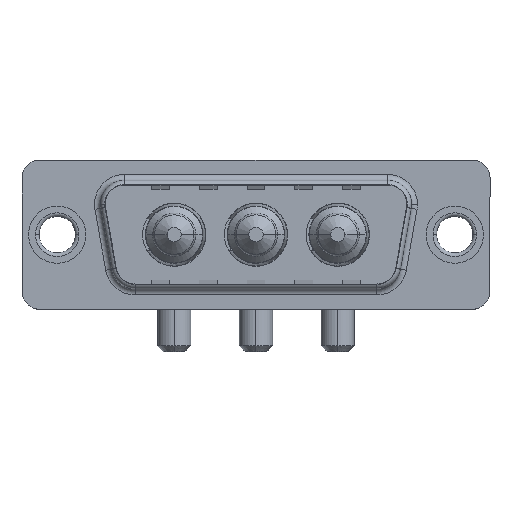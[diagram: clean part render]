
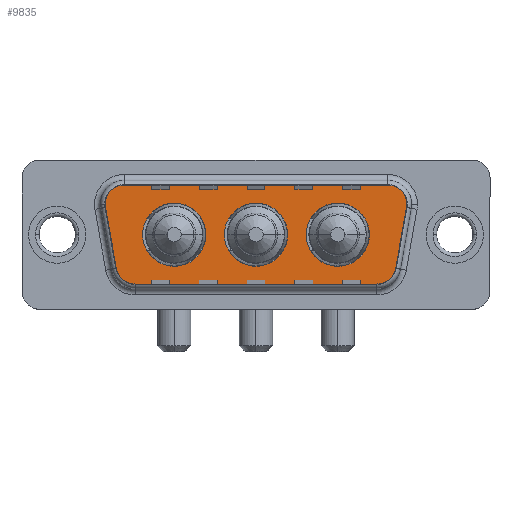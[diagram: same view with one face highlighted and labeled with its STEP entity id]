
A CAD part, top view. The second image highlights one B-rep face of the part: STEP entity #9835.
In plain terms, the highlighted planar face has unit normal (0, 0, 1).
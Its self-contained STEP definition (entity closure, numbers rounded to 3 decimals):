
#1 = ORIENTED_EDGE ( 'NONE', *, *, #4880, .F. ) ;
#44 = AXIS2_PLACEMENT_3D ( 'NONE', #7208, #10573, #5472 ) ;
#92 = AXIS2_PLACEMENT_3D ( 'NONE', #6637, #8243, #7422 ) ;
#190 = EDGE_CURVE ( 'NONE', #2033, #9514, #4935, .T. ) ;
#440 = CIRCLE ( 'NONE', #3125, 2.65 ) ;
#568 = FACE_OUTER_BOUND ( 'NONE', #8576, .T. ) ;
#621 = AXIS2_PLACEMENT_3D ( 'NONE', #5658, #1406, #4826 ) ;
#686 = VERTEX_POINT ( 'NONE', #8167 ) ;
#808 = EDGE_CURVE ( 'NONE', #7462, #11088, #4369, .T. ) ;
#855 = CARTESIAN_POINT ( 'NONE',  ( 19.3, 0., 0. ) ) ;
#932 = DIRECTION ( 'NONE',  ( 0., 0., 1. ) ) ;
#1014 = DIRECTION ( 'NONE',  ( 0., 0., 1. ) ) ;
#1162 = EDGE_CURVE ( 'NONE', #4304, #8829, #8399, .T. ) ;
#1258 = VERTEX_POINT ( 'NONE', #6361 ) ;
#1292 = ORIENTED_EDGE ( 'NONE', *, *, #190, .F. ) ;
#1401 = ORIENTED_EDGE ( 'NONE', *, *, #7856, .F. ) ;
#1406 = DIRECTION ( 'NONE',  ( 0., 0., 1. ) ) ;
#1483 = CARTESIAN_POINT ( 'NONE',  ( 27.889, 2.9, 0. ) ) ;
#1590 = VERTEX_POINT ( 'NONE', #9598 ) ;
#1840 = ORIENTED_EDGE ( 'NONE', *, *, #4806, .T. ) ;
#1907 = CARTESIAN_POINT ( 'NONE',  ( 26.866, -2.9, 0. ) ) ;
#2027 = CIRCLE ( 'NONE', #10440, 2.65 ) ;
#2033 = VERTEX_POINT ( 'NONE', #855 ) ;
#2244 = AXIS2_PLACEMENT_3D ( 'NONE', #3614, #932, #7039 ) ;
#2468 = CARTESIAN_POINT ( 'NONE',  ( 29.889, 2.9, 0. ) ) ;
#2721 = AXIS2_PLACEMENT_3D ( 'NONE', #9283, #3188, #5027 ) ;
#2795 = EDGE_CURVE ( 'NONE', #11085, #10579, #7796, .T. ) ;
#2865 = ORIENTED_EDGE ( 'NONE', *, *, #808, .T. ) ;
#2924 = ORIENTED_EDGE ( 'NONE', *, *, #4867, .T. ) ;
#3125 = AXIS2_PLACEMENT_3D ( 'NONE', #7831, #1014, #4429 ) ;
#3150 = CARTESIAN_POINT ( 'NONE',  ( 6.434, -4.9, 0. ) ) ;
#3188 = DIRECTION ( 'NONE',  ( 0., 0., 1. ) ) ;
#3232 = EDGE_LOOP ( 'NONE', ( #1, #10643 ) ) ;
#3391 = CARTESIAN_POINT ( 'NONE',  ( 26.866, -4.9, 0. ) ) ;
#3614 = CARTESIAN_POINT ( 'NONE',  ( 16.65, 0., 0. ) ) ;
#3629 = CIRCLE ( 'NONE', #9703, 2. ) ;
#3659 = CARTESIAN_POINT ( 'NONE',  ( 3.441, 2.553, 0. ) ) ;
#3798 = CARTESIAN_POINT ( 'NONE',  ( 29.859, 2.553, 0. ) ) ;
#3878 = CARTESIAN_POINT ( 'NONE',  ( 20.85, 0., 0. ) ) ;
#3948 = ORIENTED_EDGE ( 'NONE', *, *, #4537, .F. ) ;
#4004 = AXIS2_PLACEMENT_3D ( 'NONE', #1907, #10366, #7887 ) ;
#4057 = CARTESIAN_POINT ( 'NONE',  ( 14., 0., 0. ) ) ;
#4256 = LINE ( 'NONE', #5938, #7738 ) ;
#4304 = VERTEX_POINT ( 'NONE', #3878 ) ;
#4369 = LINE ( 'NONE', #10255, #5380 ) ;
#4429 = DIRECTION ( 'NONE',  ( 1., 0., 0. ) ) ;
#4433 = LINE ( 'NONE', #5432, #8589 ) ;
#4467 = CARTESIAN_POINT ( 'NONE',  ( 6.434, -2.9, 0. ) ) ;
#4537 = EDGE_CURVE ( 'NONE', #9514, #2033, #440, .T. ) ;
#4670 = DIRECTION ( 'NONE',  ( 0., 0., 1. ) ) ;
#4687 = DIRECTION ( 'NONE',  ( 0., 0., 1. ) ) ;
#4806 = EDGE_CURVE ( 'NONE', #6352, #5227, #7903, .T. ) ;
#4826 = DIRECTION ( 'NONE',  ( 1., 0., 0. ) ) ;
#4867 = EDGE_CURVE ( 'NONE', #7434, #8744, #7737, .T. ) ;
#4880 = EDGE_CURVE ( 'NONE', #8829, #4304, #8270, .T. ) ;
#4935 = CIRCLE ( 'NONE', #2244, 2.65 ) ;
#5027 = DIRECTION ( 'NONE',  ( 1., 0., 0. ) ) ;
#5227 = VERTEX_POINT ( 'NONE', #6472 ) ;
#5267 = AXIS2_PLACEMENT_3D ( 'NONE', #4467, #4687, #10472 ) ;
#5380 = VECTOR ( 'NONE', #8620, 1000. ) ;
#5432 = CARTESIAN_POINT ( 'NONE',  ( 3.441, 2.553, 0. ) ) ;
#5439 = CARTESIAN_POINT ( 'NONE',  ( 5.411, 4.9, 0. ) ) ;
#5472 = DIRECTION ( 'NONE',  ( -1., 0., 0. ) ) ;
#5593 = FACE_BOUND ( 'NONE', #10074, .T. ) ;
#5658 = CARTESIAN_POINT ( 'NONE',  ( 26.866, -2.9, 0. ) ) ;
#5938 = CARTESIAN_POINT ( 'NONE',  ( 5.411, 4.9, 0. ) ) ;
#6054 = DIRECTION ( 'NONE',  ( 0.174, -0.985, 0. ) ) ;
#6352 = VERTEX_POINT ( 'NONE', #2468 ) ;
#6361 = CARTESIAN_POINT ( 'NONE',  ( 7.15, 0., 0. ) ) ;
#6414 = DIRECTION ( 'NONE',  ( -1., 0., 0. ) ) ;
#6472 = CARTESIAN_POINT ( 'NONE',  ( 27.889, 4.9, 0. ) ) ;
#6501 = PLANE ( 'NONE',  #621 ) ;
#6580 = EDGE_CURVE ( 'NONE', #686, #11085, #8312, .T. ) ;
#6637 = CARTESIAN_POINT ( 'NONE',  ( 9.8, 0., 0. ) ) ;
#6725 = CIRCLE ( 'NONE', #92, 2.65 ) ;
#6850 = CARTESIAN_POINT ( 'NONE',  ( 6.434, -4.9, 0. ) ) ;
#6898 = VECTOR ( 'NONE', #10271, 1000. ) ;
#7039 = DIRECTION ( 'NONE',  ( 1., 0., 0. ) ) ;
#7110 = EDGE_CURVE ( 'NONE', #1590, #1258, #6725, .T. ) ;
#7168 = FACE_BOUND ( 'NONE', #3232, .T. ) ;
#7208 = CARTESIAN_POINT ( 'NONE',  ( 27.889, 2.9, 0. ) ) ;
#7422 = DIRECTION ( 'NONE',  ( 1., 0., 0. ) ) ;
#7434 = VERTEX_POINT ( 'NONE', #5439 ) ;
#7443 = DIRECTION ( 'NONE',  ( 0., 0., 1. ) ) ;
#7462 = VERTEX_POINT ( 'NONE', #8963 ) ;
#7558 = DIRECTION ( 'NONE',  ( 0., 0., 1. ) ) ;
#7608 = EDGE_CURVE ( 'NONE', #5227, #7434, #4256, .T. ) ;
#7718 = ORIENTED_EDGE ( 'NONE', *, *, #2795, .T. ) ;
#7737 = CIRCLE ( 'NONE', #8805, 2. ) ;
#7738 = VECTOR ( 'NONE', #10358, 1000. ) ;
#7796 = LINE ( 'NONE', #6850, #6898 ) ;
#7831 = CARTESIAN_POINT ( 'NONE',  ( 16.65, 0., 0. ) ) ;
#7856 = EDGE_CURVE ( 'NONE', #1258, #1590, #2027, .T. ) ;
#7887 = DIRECTION ( 'NONE',  ( 1., 0., 0. ) ) ;
#7903 = CIRCLE ( 'NONE', #44, 2. ) ;
#7913 = CARTESIAN_POINT ( 'NONE',  ( 23.5, 0., 0. ) ) ;
#7937 = ORIENTED_EDGE ( 'NONE', *, *, #7110, .F. ) ;
#8003 = FACE_BOUND ( 'NONE', #10552, .T. ) ;
#8167 = CARTESIAN_POINT ( 'NONE',  ( 4.464, -3.247, 0. ) ) ;
#8243 = DIRECTION ( 'NONE',  ( 0., 0., 1. ) ) ;
#8270 = CIRCLE ( 'NONE', #2721, 2.65 ) ;
#8312 = CIRCLE ( 'NONE', #5267, 2. ) ;
#8399 = CIRCLE ( 'NONE', #9131, 2.65 ) ;
#8401 = ORIENTED_EDGE ( 'NONE', *, *, #9734, .T. ) ;
#8576 = EDGE_LOOP ( 'NONE', ( #8401, #2865, #10884, #1840, #10947, #2924, #10266, #9241, #7718 ) ) ;
#8589 = VECTOR ( 'NONE', #6054, 1000. ) ;
#8620 = DIRECTION ( 'NONE',  ( 0.174, 0.985, 0. ) ) ;
#8744 = VERTEX_POINT ( 'NONE', #3659 ) ;
#8781 = DIRECTION ( 'NONE',  ( 1., 0., 0. ) ) ;
#8805 = AXIS2_PLACEMENT_3D ( 'NONE', #9237, #7443, #10022 ) ;
#8820 = CIRCLE ( 'NONE', #4004, 2. ) ;
#8829 = VERTEX_POINT ( 'NONE', #10044 ) ;
#8953 = EDGE_CURVE ( 'NONE', #11088, #6352, #3629, .T. ) ;
#8963 = CARTESIAN_POINT ( 'NONE',  ( 28.836, -3.247, 0. ) ) ;
#9131 = AXIS2_PLACEMENT_3D ( 'NONE', #7913, #7558, #10188 ) ;
#9237 = CARTESIAN_POINT ( 'NONE',  ( 5.411, 2.9, 0. ) ) ;
#9241 = ORIENTED_EDGE ( 'NONE', *, *, #6580, .T. ) ;
#9283 = CARTESIAN_POINT ( 'NONE',  ( 23.5, 0., 0. ) ) ;
#9514 = VERTEX_POINT ( 'NONE', #4057 ) ;
#9598 = CARTESIAN_POINT ( 'NONE',  ( 12.45, 0., 0. ) ) ;
#9671 = CARTESIAN_POINT ( 'NONE',  ( 9.8, 0., 0. ) ) ;
#9703 = AXIS2_PLACEMENT_3D ( 'NONE', #1483, #4670, #6414 ) ;
#9734 = EDGE_CURVE ( 'NONE', #10579, #7462, #8820, .T. ) ;
#9835 = ADVANCED_FACE ( 'NONE', ( #5593, #7168, #8003, #568 ), #6501, .T. ) ;
#10022 = DIRECTION ( 'NONE',  ( 1., 0., 0. ) ) ;
#10044 = CARTESIAN_POINT ( 'NONE',  ( 26.15, 0., 0. ) ) ;
#10074 = EDGE_LOOP ( 'NONE', ( #1292, #3948 ) ) ;
#10188 = DIRECTION ( 'NONE',  ( 1., 0., 0. ) ) ;
#10255 = CARTESIAN_POINT ( 'NONE',  ( 29.859, 2.553, 0. ) ) ;
#10266 = ORIENTED_EDGE ( 'NONE', *, *, #10978, .T. ) ;
#10271 = DIRECTION ( 'NONE',  ( 1., 0., 0. ) ) ;
#10358 = DIRECTION ( 'NONE',  ( -1., 0., 0. ) ) ;
#10366 = DIRECTION ( 'NONE',  ( 0., 0., 1. ) ) ;
#10440 = AXIS2_PLACEMENT_3D ( 'NONE', #9671, #10644, #8781 ) ;
#10472 = DIRECTION ( 'NONE',  ( -1., 0., 0. ) ) ;
#10552 = EDGE_LOOP ( 'NONE', ( #7937, #1401 ) ) ;
#10573 = DIRECTION ( 'NONE',  ( 0., 0., 1. ) ) ;
#10579 = VERTEX_POINT ( 'NONE', #3391 ) ;
#10643 = ORIENTED_EDGE ( 'NONE', *, *, #1162, .F. ) ;
#10644 = DIRECTION ( 'NONE',  ( 0., 0., 1. ) ) ;
#10884 = ORIENTED_EDGE ( 'NONE', *, *, #8953, .T. ) ;
#10947 = ORIENTED_EDGE ( 'NONE', *, *, #7608, .T. ) ;
#10978 = EDGE_CURVE ( 'NONE', #8744, #686, #4433, .T. ) ;
#11085 = VERTEX_POINT ( 'NONE', #3150 ) ;
#11088 = VERTEX_POINT ( 'NONE', #3798 ) ;
